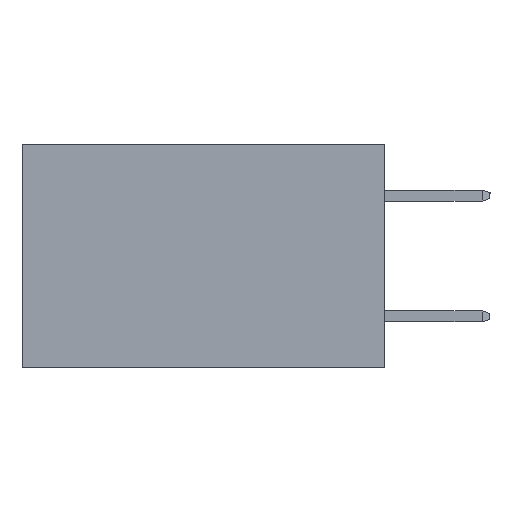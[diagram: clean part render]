
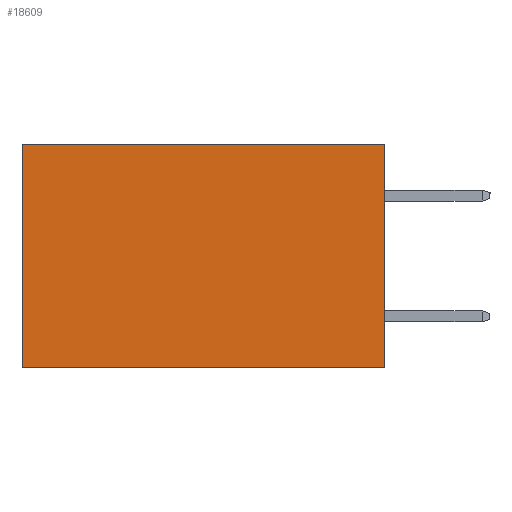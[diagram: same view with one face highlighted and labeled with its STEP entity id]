
A CAD part, left-side view. The second image highlights one B-rep face of the part: STEP entity #18609.
In plain terms, the highlighted planar face has unit normal (-1, 0, 0).
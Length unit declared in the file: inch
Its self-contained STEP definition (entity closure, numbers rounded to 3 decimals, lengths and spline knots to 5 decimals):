
#521 = ORIENTED_EDGE ( 'NONE', *, *, #7256, .F. ) ;
#2636 = VERTEX_POINT ( 'NONE', #15591 ) ;
#2729 = DIRECTION ( 'NONE',  ( 0., 1., 0. ) ) ;
#3019 = VECTOR ( 'NONE', #19105, 39.37008 ) ;
#3169 = CARTESIAN_POINT ( 'NONE',  ( 0.2615, 0., -0.37 ) ) ;
#3563 = VERTEX_POINT ( 'NONE', #10780 ) ;
#3739 = VECTOR ( 'NONE', #20081, 39.37008 ) ;
#7256 = EDGE_CURVE ( 'NONE', #9955, #2636, #7527, .T. ) ;
#7323 = ORIENTED_EDGE ( 'NONE', *, *, #10098, .T. ) ;
#7527 = LINE ( 'NONE', #3169, #3019 ) ;
#7797 = FACE_OUTER_BOUND ( 'NONE', #13188, .T. ) ;
#8001 = VECTOR ( 'NONE', #2729, 39.37008 ) ;
#8367 = CARTESIAN_POINT ( 'NONE',  ( 0.2615, 0.6, -0.37 ) ) ;
#9263 = ORIENTED_EDGE ( 'NONE', *, *, #12208, .F. ) ;
#9925 = LINE ( 'NONE', #8367, #11108 ) ;
#9955 = VERTEX_POINT ( 'NONE', #14693 ) ;
#10098 = EDGE_CURVE ( 'NONE', #9955, #11712, #10673, .T. ) ;
#10673 = LINE ( 'NONE', #19822, #8001 ) ;
#10780 = CARTESIAN_POINT ( 'NONE',  ( 0.2615, 0.6, -0.37 ) ) ;
#11108 = VECTOR ( 'NONE', #15493, 39.37008 ) ;
#11712 = VERTEX_POINT ( 'NONE', #13119 ) ;
#11951 = ORIENTED_EDGE ( 'NONE', *, *, #13708, .T. ) ;
#12208 = EDGE_CURVE ( 'NONE', #2636, #3563, #13682, .T. ) ;
#12758 = DIRECTION ( 'NONE',  ( 1., 0., 0. ) ) ;
#13119 = CARTESIAN_POINT ( 'NONE',  ( 0.2615, 0.6, 0. ) ) ;
#13188 = EDGE_LOOP ( 'NONE', ( #11951, #9263, #521, #7323 ) ) ;
#13568 = CARTESIAN_POINT ( 'NONE',  ( 0.2615, 0., -0.37 ) ) ;
#13682 = LINE ( 'NONE', #13568, #3739 ) ;
#13708 = EDGE_CURVE ( 'NONE', #11712, #3563, #9925, .T. ) ;
#14313 = DIRECTION ( 'NONE',  ( 0., 0., -1. ) ) ;
#14693 = CARTESIAN_POINT ( 'NONE',  ( 0.2615, 0., 0. ) ) ;
#14896 = AXIS2_PLACEMENT_3D ( 'NONE', #19267, #12758, #14313 ) ;
#15493 = DIRECTION ( 'NONE',  ( 0., 0., -1. ) ) ;
#15572 = PLANE ( 'NONE',  #14896 ) ;
#15591 = CARTESIAN_POINT ( 'NONE',  ( 0.2615, 0., -0.37 ) ) ;
#18609 = ADVANCED_FACE ( 'NONE', ( #7797 ), #15572, .F. ) ;
#19105 = DIRECTION ( 'NONE',  ( 0., 0., -1. ) ) ;
#19267 = CARTESIAN_POINT ( 'NONE',  ( 0.2615, 0., -0.37 ) ) ;
#19822 = CARTESIAN_POINT ( 'NONE',  ( 0.2615, 0., 0. ) ) ;
#20081 = DIRECTION ( 'NONE',  ( 0., 1., 0. ) ) ;
